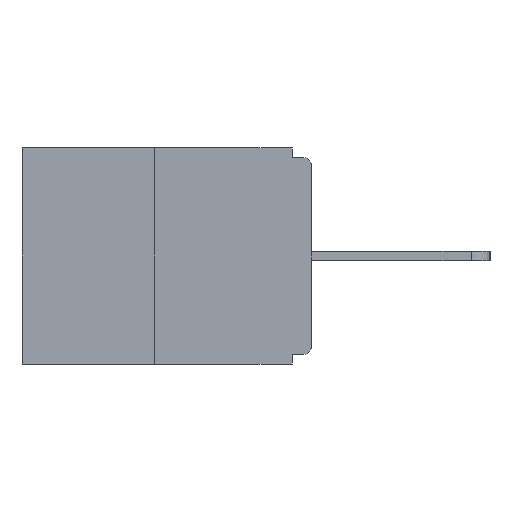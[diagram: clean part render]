
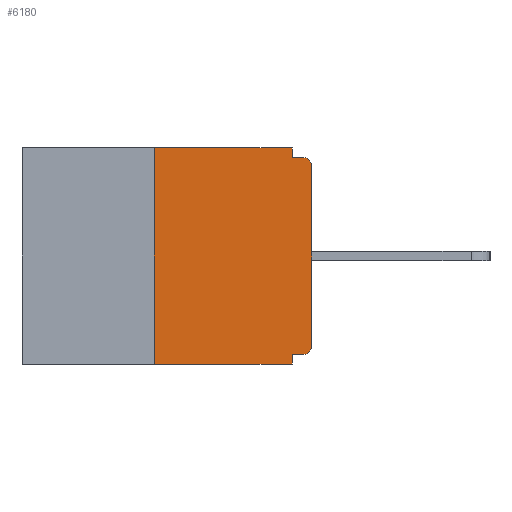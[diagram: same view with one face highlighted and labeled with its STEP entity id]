
A CAD part, left-side view. The second image highlights one B-rep face of the part: STEP entity #6180.
In plain terms, the highlighted planar face has unit normal (-1, 0, 0).
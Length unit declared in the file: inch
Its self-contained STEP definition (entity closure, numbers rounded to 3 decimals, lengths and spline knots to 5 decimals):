
#431 = DIRECTION ( 'NONE',  ( 0., 0., -1. ) ) ;
#536 = LINE ( 'NONE', #14394, #12478 ) ;
#635 = EDGE_CURVE ( 'NONE', #9917, #3217, #8966, .T. ) ;
#758 = CARTESIAN_POINT ( 'NONE',  ( 0., 0., -0.328 ) ) ;
#820 = DIRECTION ( 'NONE',  ( -1., 0., 0. ) ) ;
#1017 = LINE ( 'NONE', #7143, #7463 ) ;
#1062 = CARTESIAN_POINT ( 'NONE',  ( 0., 0., -0.03 ) ) ;
#1069 = ORIENTED_EDGE ( 'NONE', *, *, #13236, .F. ) ;
#1441 = CARTESIAN_POINT ( 'NONE',  ( 0., 0.25, -0.343 ) ) ;
#1469 = DIRECTION ( 'NONE',  ( 0., -1., 0. ) ) ;
#1538 = AXIS2_PLACEMENT_3D ( 'NONE', #4087, #12461, #14785 ) ;
#1729 = EDGE_CURVE ( 'NONE', #5877, #3107, #1017, .T. ) ;
#1921 = ORIENTED_EDGE ( 'NONE', *, *, #7246, .F. ) ;
#2043 = DIRECTION ( 'NONE',  ( 0., 0., -1. ) ) ;
#2101 = CARTESIAN_POINT ( 'NONE',  ( 0., 0.031, -0.328 ) ) ;
#2459 = LINE ( 'NONE', #758, #9830 ) ;
#2464 = VERTEX_POINT ( 'NONE', #9711 ) ;
#2588 = ORIENTED_EDGE ( 'NONE', *, *, #9897, .T. ) ;
#2680 = EDGE_CURVE ( 'NONE', #6229, #13461, #2459, .T. ) ;
#2688 = EDGE_CURVE ( 'NONE', #2464, #9917, #10921, .T. ) ;
#2986 = DIRECTION ( 'NONE',  ( 1., 0., 0. ) ) ;
#3107 = VERTEX_POINT ( 'NONE', #1062 ) ;
#3217 = VERTEX_POINT ( 'NONE', #8278 ) ;
#3265 = VECTOR ( 'NONE', #431, 39.37008 ) ;
#3359 = EDGE_CURVE ( 'NONE', #3217, #10199, #7418, .T. ) ;
#3587 = DIRECTION ( 'NONE',  ( 0., 0., 1. ) ) ;
#3832 = ORIENTED_EDGE ( 'NONE', *, *, #2688, .F. ) ;
#3956 = ORIENTED_EDGE ( 'NONE', *, *, #635, .F. ) ;
#4005 = LINE ( 'NONE', #9953, #3265 ) ;
#4039 = CIRCLE ( 'NONE', #6486, 0.015 ) ;
#4087 = CARTESIAN_POINT ( 'NONE',  ( 0., 0.015, -0.03 ) ) ;
#4286 = CARTESIAN_POINT ( 'NONE',  ( 0., 0.031, 0. ) ) ;
#4658 = CIRCLE ( 'NONE', #1538, 0.015 ) ;
#5088 = DIRECTION ( 'NONE',  ( 0., 0., 1. ) ) ;
#5572 = CARTESIAN_POINT ( 'NONE',  ( 0., 0.015, -0.313 ) ) ;
#5712 = DIRECTION ( 'NONE',  ( 0., -1., 0. ) ) ;
#5813 = CARTESIAN_POINT ( 'NONE',  ( 0., 0.46, 0. ) ) ;
#5877 = VERTEX_POINT ( 'NONE', #5975 ) ;
#5975 = CARTESIAN_POINT ( 'NONE',  ( 0., 0., -0.313 ) ) ;
#5984 = ORIENTED_EDGE ( 'NONE', *, *, #15091, .T. ) ;
#6153 = FACE_OUTER_BOUND ( 'NONE', #13423, .T. ) ;
#6180 = ADVANCED_FACE ( 'NONE', ( #6153 ), #8869, .F. ) ;
#6229 = VERTEX_POINT ( 'NONE', #14565 ) ;
#6341 = DIRECTION ( 'NONE',  ( 0., -1., 0. ) ) ;
#6429 = ORIENTED_EDGE ( 'NONE', *, *, #15226, .T. ) ;
#6486 = AXIS2_PLACEMENT_3D ( 'NONE', #5572, #820, #2043 ) ;
#6861 = VERTEX_POINT ( 'NONE', #1441 ) ;
#7143 = CARTESIAN_POINT ( 'NONE',  ( 0., 0., 0. ) ) ;
#7246 = EDGE_CURVE ( 'NONE', #6861, #2464, #536, .T. ) ;
#7418 = LINE ( 'NONE', #13267, #13279 ) ;
#7463 = VECTOR ( 'NONE', #3587, 39.37008 ) ;
#8278 = CARTESIAN_POINT ( 'NONE',  ( 0., 0.031, -0.015 ) ) ;
#8775 = CARTESIAN_POINT ( 'NONE',  ( 0., 0.46, -0.343 ) ) ;
#8869 = PLANE ( 'NONE',  #10224 ) ;
#8966 = LINE ( 'NONE', #4286, #11171 ) ;
#9044 = CARTESIAN_POINT ( 'NONE',  ( 0., 0.031, 0. ) ) ;
#9711 = CARTESIAN_POINT ( 'NONE',  ( 0., 0.25, 0. ) ) ;
#9830 = VECTOR ( 'NONE', #15227, 39.37008 ) ;
#9897 = EDGE_CURVE ( 'NONE', #6229, #5877, #4039, .T. ) ;
#9917 = VERTEX_POINT ( 'NONE', #9044 ) ;
#9953 = CARTESIAN_POINT ( 'NONE',  ( 0., 0.031, -0.343 ) ) ;
#10050 = CARTESIAN_POINT ( 'NONE',  ( 0., 0.46, 0. ) ) ;
#10196 = LINE ( 'NONE', #8775, #12564 ) ;
#10199 = VERTEX_POINT ( 'NONE', #14683 ) ;
#10224 = AXIS2_PLACEMENT_3D ( 'NONE', #10050, #2986, #11217 ) ;
#10449 = ORIENTED_EDGE ( 'NONE', *, *, #3359, .F. ) ;
#10736 = CARTESIAN_POINT ( 'NONE',  ( 0., 0.031, -0.343 ) ) ;
#10921 = LINE ( 'NONE', #5813, #13644 ) ;
#11171 = VECTOR ( 'NONE', #11241, 39.37008 ) ;
#11217 = DIRECTION ( 'NONE',  ( 0., 0., -1. ) ) ;
#11241 = DIRECTION ( 'NONE',  ( 0., 0., -1. ) ) ;
#12461 = DIRECTION ( 'NONE',  ( -1., 0., 0. ) ) ;
#12478 = VECTOR ( 'NONE', #5088, 39.37008 ) ;
#12564 = VECTOR ( 'NONE', #6341, 39.37008 ) ;
#13236 = EDGE_CURVE ( 'NONE', #13461, #13984, #4005, .T. ) ;
#13267 = CARTESIAN_POINT ( 'NONE',  ( 0., 0., -0.015 ) ) ;
#13279 = VECTOR ( 'NONE', #1469, 39.37008 ) ;
#13423 = EDGE_LOOP ( 'NONE', ( #3832, #1921, #5984, #1069, #14877, #2588, #14685, #6429, #10449, #3956 ) ) ;
#13461 = VERTEX_POINT ( 'NONE', #2101 ) ;
#13644 = VECTOR ( 'NONE', #5712, 39.37008 ) ;
#13984 = VERTEX_POINT ( 'NONE', #10736 ) ;
#14394 = CARTESIAN_POINT ( 'NONE',  ( 0., 0.25, 0. ) ) ;
#14565 = CARTESIAN_POINT ( 'NONE',  ( 0., 0.015, -0.328 ) ) ;
#14683 = CARTESIAN_POINT ( 'NONE',  ( 0., 0.015, -0.015 ) ) ;
#14685 = ORIENTED_EDGE ( 'NONE', *, *, #1729, .T. ) ;
#14785 = DIRECTION ( 'NONE',  ( 0., 0., -1. ) ) ;
#14877 = ORIENTED_EDGE ( 'NONE', *, *, #2680, .F. ) ;
#15091 = EDGE_CURVE ( 'NONE', #6861, #13984, #10196, .T. ) ;
#15226 = EDGE_CURVE ( 'NONE', #3107, #10199, #4658, .T. ) ;
#15227 = DIRECTION ( 'NONE',  ( 0., 1., 0. ) ) ;
